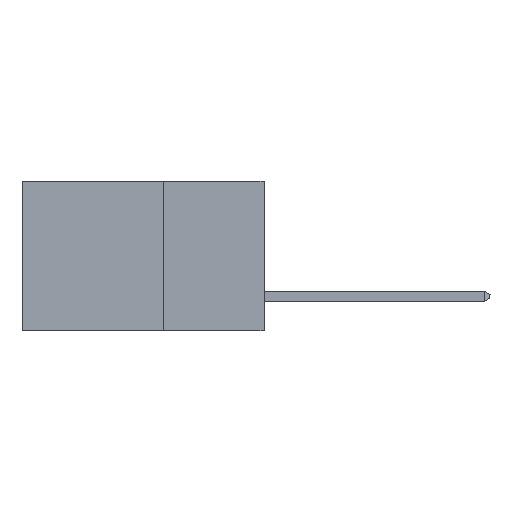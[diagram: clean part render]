
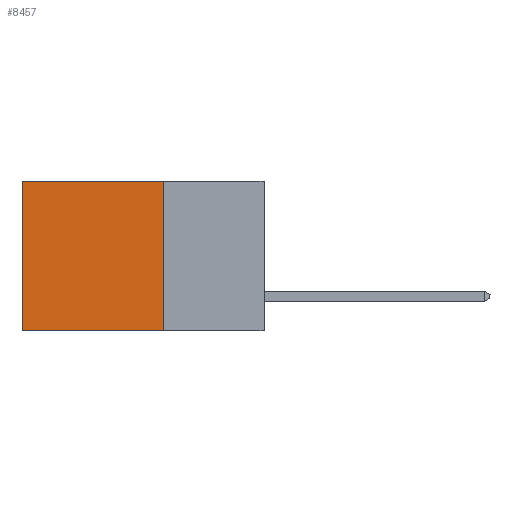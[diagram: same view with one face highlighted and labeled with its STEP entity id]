
A CAD part, left-side view. The second image highlights one B-rep face of the part: STEP entity #8457.
In plain terms, the highlighted planar face has unit normal (-1, 0, 0).
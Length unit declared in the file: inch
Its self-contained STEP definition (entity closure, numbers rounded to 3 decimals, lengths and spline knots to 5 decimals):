
#797 = EDGE_CURVE ( 'NONE', #19137, #18309, #9100, .T. ) ;
#806 = CARTESIAN_POINT ( 'NONE',  ( 0.2615, 0.25, -0.37 ) ) ;
#1801 = VERTEX_POINT ( 'NONE', #6473 ) ;
#2450 = ORIENTED_EDGE ( 'NONE', *, *, #21209, .F. ) ;
#2787 = ORIENTED_EDGE ( 'NONE', *, *, #6817, .T. ) ;
#3322 = CARTESIAN_POINT ( 'NONE',  ( 0.2615, 0.6, -0.37 ) ) ;
#3921 = CARTESIAN_POINT ( 'NONE',  ( 0.2615, 0.25, -0.37 ) ) ;
#4454 = DIRECTION ( 'NONE',  ( 0., 0., -1. ) ) ;
#5181 = VECTOR ( 'NONE', #5320, 39.37008 ) ;
#5320 = DIRECTION ( 'NONE',  ( 0., 0., -1. ) ) ;
#5515 = LINE ( 'NONE', #23366, #15779 ) ;
#5544 = CARTESIAN_POINT ( 'NONE',  ( 0.2615, 0.25, -0.37 ) ) ;
#5632 = DIRECTION ( 'NONE',  ( 0., 1., 0. ) ) ;
#5857 = CARTESIAN_POINT ( 'NONE',  ( 0.2615, 0.6, 0. ) ) ;
#5913 = DIRECTION ( 'NONE',  ( 0., 0., -1. ) ) ;
#5964 = CARTESIAN_POINT ( 'NONE',  ( 0.2615, 0.25, 0. ) ) ;
#6003 = DIRECTION ( 'NONE',  ( 0., 1., 0. ) ) ;
#6280 = AXIS2_PLACEMENT_3D ( 'NONE', #3921, #17449, #5913 ) ;
#6473 = CARTESIAN_POINT ( 'NONE',  ( 0.2615, 0.25, 0. ) ) ;
#6817 = EDGE_CURVE ( 'NONE', #1801, #6824, #24009, .T. ) ;
#6824 = VERTEX_POINT ( 'NONE', #5857 ) ;
#8457 = ADVANCED_FACE ( 'NONE', ( #12651 ), #15537, .F. ) ;
#8494 = VECTOR ( 'NONE', #5632, 39.37008 ) ;
#9100 = LINE ( 'NONE', #5544, #8494 ) ;
#11178 = ORIENTED_EDGE ( 'NONE', *, *, #21426, .T. ) ;
#12651 = FACE_OUTER_BOUND ( 'NONE', #19297, .T. ) ;
#14862 = ORIENTED_EDGE ( 'NONE', *, *, #797, .F. ) ;
#15465 = LINE ( 'NONE', #3322, #5181 ) ;
#15537 = PLANE ( 'NONE',  #6280 ) ;
#15779 = VECTOR ( 'NONE', #4454, 39.37008 ) ;
#17449 = DIRECTION ( 'NONE',  ( 1., 0., 0. ) ) ;
#17638 = CARTESIAN_POINT ( 'NONE',  ( 0.2615, 0.6, -0.37 ) ) ;
#18309 = VERTEX_POINT ( 'NONE', #17638 ) ;
#19137 = VERTEX_POINT ( 'NONE', #806 ) ;
#19277 = VECTOR ( 'NONE', #6003, 39.37008 ) ;
#19297 = EDGE_LOOP ( 'NONE', ( #11178, #14862, #2450, #2787 ) ) ;
#21209 = EDGE_CURVE ( 'NONE', #1801, #19137, #5515, .T. ) ;
#21426 = EDGE_CURVE ( 'NONE', #6824, #18309, #15465, .T. ) ;
#23366 = CARTESIAN_POINT ( 'NONE',  ( 0.2615, 0.25, -0.37 ) ) ;
#24009 = LINE ( 'NONE', #5964, #19277 ) ;
